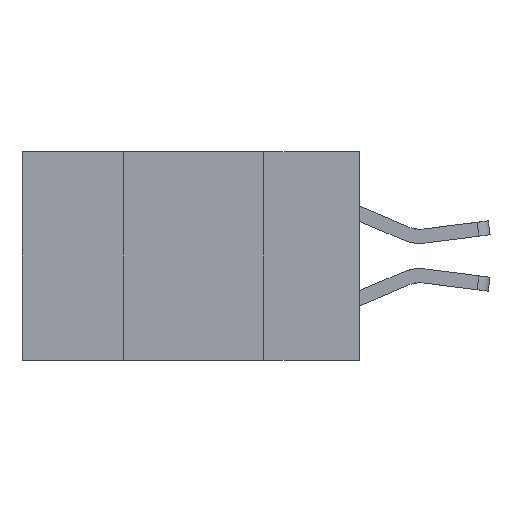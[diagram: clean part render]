
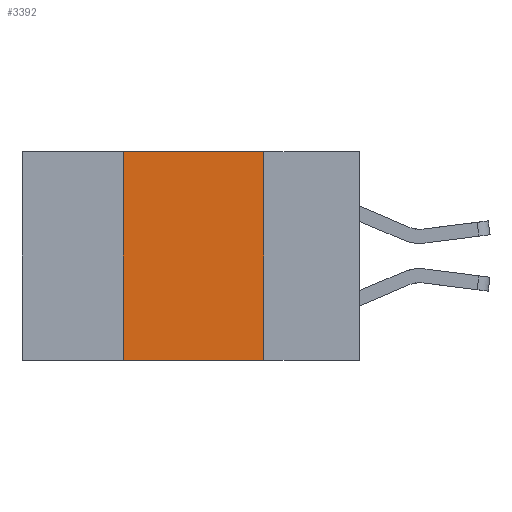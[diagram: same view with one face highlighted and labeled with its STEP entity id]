
A CAD part, left-side view. The second image highlights one B-rep face of the part: STEP entity #3392.
In plain terms, the highlighted planar face has unit normal (-1, 0, 0).
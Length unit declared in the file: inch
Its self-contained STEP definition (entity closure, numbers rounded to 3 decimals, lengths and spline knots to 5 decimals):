
#284 = PLANE ( 'NONE',  #529 ) ;
#386 = FACE_OUTER_BOUND ( 'NONE', #642, .T. ) ;
#529 = AXIS2_PLACEMENT_3D ( 'NONE', #1927, #5240, #7513 ) ;
#642 = EDGE_LOOP ( 'NONE', ( #9008, #10269, #1217, #3458 ) ) ;
#1217 = ORIENTED_EDGE ( 'NONE', *, *, #5238, .F. ) ;
#1527 = DIRECTION ( 'NONE',  ( 0., -1., 0. ) ) ;
#1927 = CARTESIAN_POINT ( 'NONE',  ( 0., 0.6, 0. ) ) ;
#2112 = DIRECTION ( 'NONE',  ( 0., -1., 0. ) ) ;
#2267 = LINE ( 'NONE', #4587, #9857 ) ;
#3392 = ADVANCED_FACE ( 'NONE', ( #386 ), #284, .F. ) ;
#3458 = ORIENTED_EDGE ( 'NONE', *, *, #9753, .T. ) ;
#3540 = LINE ( 'NONE', #6720, #8398 ) ;
#4393 = CARTESIAN_POINT ( 'NONE',  ( 0., 0.42, 0. ) ) ;
#4587 = CARTESIAN_POINT ( 'NONE',  ( 0., 0.6, -0.37 ) ) ;
#5001 = VERTEX_POINT ( 'NONE', #6290 ) ;
#5040 = EDGE_CURVE ( 'NONE', #7837, #5001, #8812, .T. ) ;
#5238 = EDGE_CURVE ( 'NONE', #9778, #7837, #3540, .T. ) ;
#5240 = DIRECTION ( 'NONE',  ( 1., 0., 0. ) ) ;
#6290 = CARTESIAN_POINT ( 'NONE',  ( 0., 0.17, 0. ) ) ;
#6302 = LINE ( 'NONE', #7192, #7066 ) ;
#6664 = EDGE_CURVE ( 'NONE', #5001, #9519, #6302, .T. ) ;
#6695 = VECTOR ( 'NONE', #1527, 39.37008 ) ;
#6720 = CARTESIAN_POINT ( 'NONE',  ( 0., 0.42, 0. ) ) ;
#7066 = VECTOR ( 'NONE', #9509, 39.37008 ) ;
#7192 = CARTESIAN_POINT ( 'NONE',  ( 0., 0.17, 0. ) ) ;
#7513 = DIRECTION ( 'NONE',  ( 0., 0., -1. ) ) ;
#7837 = VERTEX_POINT ( 'NONE', #4393 ) ;
#8177 = CARTESIAN_POINT ( 'NONE',  ( 0., 0.17, -0.37 ) ) ;
#8398 = VECTOR ( 'NONE', #9099, 39.37008 ) ;
#8615 = CARTESIAN_POINT ( 'NONE',  ( 0., 0.6, 0. ) ) ;
#8812 = LINE ( 'NONE', #8615, #6695 ) ;
#9008 = ORIENTED_EDGE ( 'NONE', *, *, #6664, .F. ) ;
#9099 = DIRECTION ( 'NONE',  ( 0., 0., 1. ) ) ;
#9392 = CARTESIAN_POINT ( 'NONE',  ( 0., 0.42, -0.37 ) ) ;
#9509 = DIRECTION ( 'NONE',  ( 0., 0., -1. ) ) ;
#9519 = VERTEX_POINT ( 'NONE', #8177 ) ;
#9753 = EDGE_CURVE ( 'NONE', #9778, #9519, #2267, .T. ) ;
#9778 = VERTEX_POINT ( 'NONE', #9392 ) ;
#9857 = VECTOR ( 'NONE', #2112, 39.37008 ) ;
#10269 = ORIENTED_EDGE ( 'NONE', *, *, #5040, .F. ) ;
